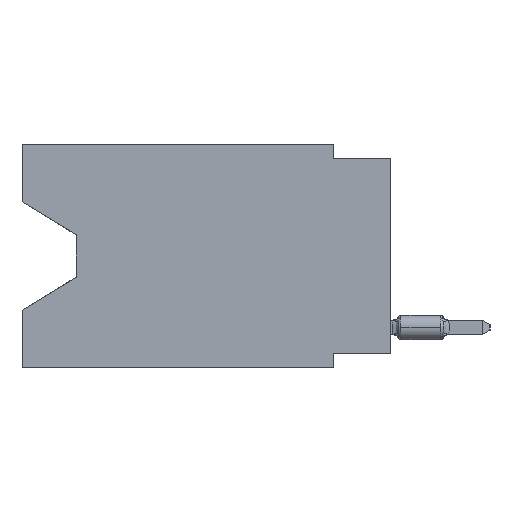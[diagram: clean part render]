
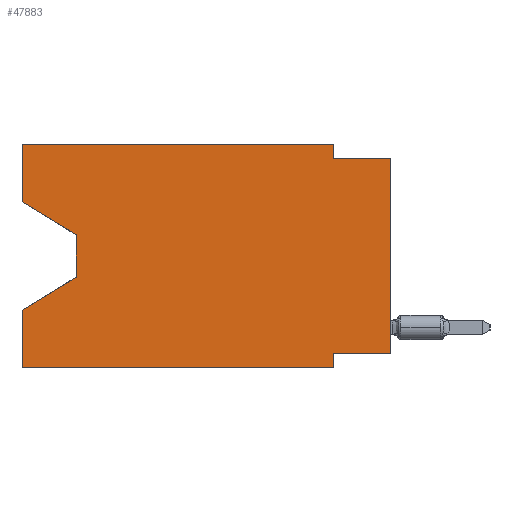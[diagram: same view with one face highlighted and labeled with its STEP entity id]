
A CAD part, left-side view. The second image highlights one B-rep face of the part: STEP entity #47883.
In plain terms, the highlighted planar face has unit normal (-1, 0, 0).
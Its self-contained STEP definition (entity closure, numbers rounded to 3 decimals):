
#1204 = CARTESIAN_POINT ( 'NONE',  ( 0., 16.383, -2.546 ) ) ;
#3223 = CARTESIAN_POINT ( 'NONE',  ( 0., 16.383, -9.906 ) ) ;
#3280 = ORIENTED_EDGE ( 'NONE', *, *, #9359, .F. ) ;
#3339 = CARTESIAN_POINT ( 'NONE',  ( 0., 16.383, 0. ) ) ;
#3977 = VERTEX_POINT ( 'NONE', #37726 ) ;
#4038 = CARTESIAN_POINT ( 'NONE',  ( 0., 0., -0.635 ) ) ;
#4689 = ORIENTED_EDGE ( 'NONE', *, *, #19832, .F. ) ;
#5137 = LINE ( 'NONE', #14670, #37281 ) ;
#5842 = AXIS2_PLACEMENT_3D ( 'NONE', #3339, #15400, #18694 ) ;
#6745 = VECTOR ( 'NONE', #31035, 1000. ) ;
#6858 = CARTESIAN_POINT ( 'NONE',  ( 0., 16.383, 0. ) ) ;
#7104 = DIRECTION ( 'NONE',  ( 0., -1., 0. ) ) ;
#7343 = LINE ( 'NONE', #22481, #6745 ) ;
#8064 = VECTOR ( 'NONE', #26135, 1000. ) ;
#8374 = EDGE_CURVE ( 'NONE', #20429, #22613, #20803, .T. ) ;
#8928 = EDGE_CURVE ( 'NONE', #46024, #38922, #5137, .T. ) ;
#9132 = EDGE_CURVE ( 'NONE', #48511, #3977, #7343, .T. ) ;
#9359 = EDGE_CURVE ( 'NONE', #46024, #48511, #25212, .T. ) ;
#10080 = EDGE_CURVE ( 'NONE', #17925, #31157, #37848, .T. ) ;
#11114 = FACE_OUTER_BOUND ( 'NONE', #37714, .T. ) ;
#11973 = CARTESIAN_POINT ( 'NONE',  ( 0., 16.383, -2.546 ) ) ;
#12024 = LINE ( 'NONE', #38232, #37107 ) ;
#12981 = CARTESIAN_POINT ( 'NONE',  ( 0., 16.383, -9.906 ) ) ;
#13785 = LINE ( 'NONE', #40510, #45194 ) ;
#14670 = CARTESIAN_POINT ( 'NONE',  ( 0., 0., 0. ) ) ;
#15400 = DIRECTION ( 'NONE',  ( 1., 0., 0. ) ) ;
#15571 = CARTESIAN_POINT ( 'NONE',  ( 0., 16.383, 0. ) ) ;
#15615 = ORIENTED_EDGE ( 'NONE', *, *, #24946, .F. ) ;
#17768 = LINE ( 'NONE', #21801, #44777 ) ;
#17925 = VERTEX_POINT ( 'NONE', #43346 ) ;
#17985 = ORIENTED_EDGE ( 'NONE', *, *, #48551, .T. ) ;
#18386 = ORIENTED_EDGE ( 'NONE', *, *, #9132, .F. ) ;
#18694 = DIRECTION ( 'NONE',  ( 0., 0., -1. ) ) ;
#18767 = VECTOR ( 'NONE', #47257, 1000. ) ;
#18847 = DIRECTION ( 'NONE',  ( 0., 0., 1. ) ) ;
#19832 = EDGE_CURVE ( 'NONE', #28555, #35747, #12024, .T. ) ;
#20429 = VERTEX_POINT ( 'NONE', #11973 ) ;
#20803 = LINE ( 'NONE', #1204, #18767 ) ;
#21218 = ORIENTED_EDGE ( 'NONE', *, *, #31844, .T. ) ;
#21319 = CARTESIAN_POINT ( 'NONE',  ( 0., 0., -0.635 ) ) ;
#21801 = CARTESIAN_POINT ( 'NONE',  ( 0., 2.54, 0. ) ) ;
#21937 = DIRECTION ( 'NONE',  ( 0., 1., 0. ) ) ;
#22116 = ORIENTED_EDGE ( 'NONE', *, *, #36524, .T. ) ;
#22481 = CARTESIAN_POINT ( 'NONE',  ( 0., 2.54, -9.906 ) ) ;
#22613 = VERTEX_POINT ( 'NONE', #39816 ) ;
#22615 = LINE ( 'NONE', #37974, #8064 ) ;
#24548 = VERTEX_POINT ( 'NONE', #49396 ) ;
#24885 = CARTESIAN_POINT ( 'NONE',  ( 0., 2.54, 0. ) ) ;
#24946 = EDGE_CURVE ( 'NONE', #20429, #17925, #37999, .T. ) ;
#25212 = LINE ( 'NONE', #40587, #38139 ) ;
#25267 = DIRECTION ( 'NONE',  ( 0., 0., 1. ) ) ;
#26135 = DIRECTION ( 'NONE',  ( 0., 0.855, -0.519 ) ) ;
#26741 = PLANE ( 'NONE',  #5842 ) ;
#27827 = DIRECTION ( 'NONE',  ( 0., 0., 1. ) ) ;
#28160 = DIRECTION ( 'NONE',  ( 0., 0., -1. ) ) ;
#28222 = VECTOR ( 'NONE', #48020, 1000. ) ;
#28357 = DIRECTION ( 'NONE',  ( 0., -1., 0. ) ) ;
#28472 = CARTESIAN_POINT ( 'NONE',  ( 0., 16.383, -7.36 ) ) ;
#28555 = VERTEX_POINT ( 'NONE', #3223 ) ;
#28644 = VECTOR ( 'NONE', #28357, 1000. ) ;
#30017 = EDGE_CURVE ( 'NONE', #31284, #38922, #48263, .T. ) ;
#31035 = DIRECTION ( 'NONE',  ( 0., 0., -1. ) ) ;
#31157 = VERTEX_POINT ( 'NONE', #24885 ) ;
#31284 = VERTEX_POINT ( 'NONE', #45287 ) ;
#31829 = ORIENTED_EDGE ( 'NONE', *, *, #30017, .F. ) ;
#31844 = EDGE_CURVE ( 'NONE', #24548, #35747, #22615, .T. ) ;
#33018 = ORIENTED_EDGE ( 'NONE', *, *, #8928, .T. ) ;
#35091 = CARTESIAN_POINT ( 'NONE',  ( 0., 0., -9.271 ) ) ;
#35747 = VERTEX_POINT ( 'NONE', #28472 ) ;
#36524 = EDGE_CURVE ( 'NONE', #28555, #3977, #43000, .T. ) ;
#36710 = EDGE_CURVE ( 'NONE', #31157, #31284, #17768, .T. ) ;
#36860 = ORIENTED_EDGE ( 'NONE', *, *, #36710, .F. ) ;
#37107 = VECTOR ( 'NONE', #18847, 1000. ) ;
#37146 = VECTOR ( 'NONE', #7104, 1000. ) ;
#37281 = VECTOR ( 'NONE', #25267, 1000. ) ;
#37714 = EDGE_LOOP ( 'NONE', ( #48249, #17985, #21218, #4689, #22116, #18386, #3280, #33018, #31829, #36860, #40764, #15615 ) ) ;
#37726 = CARTESIAN_POINT ( 'NONE',  ( 0., 2.54, -9.906 ) ) ;
#37848 = LINE ( 'NONE', #6858, #37146 ) ;
#37974 = CARTESIAN_POINT ( 'NONE',  ( 0., 13.97, -5.893 ) ) ;
#37999 = LINE ( 'NONE', #15571, #47140 ) ;
#38139 = VECTOR ( 'NONE', #21937, 1000. ) ;
#38232 = CARTESIAN_POINT ( 'NONE',  ( 0., 16.383, 0. ) ) ;
#38922 = VERTEX_POINT ( 'NONE', #4038 ) ;
#39816 = CARTESIAN_POINT ( 'NONE',  ( 0., 13.97, -4.013 ) ) ;
#40510 = CARTESIAN_POINT ( 'NONE',  ( 0., 13.97, -4.013 ) ) ;
#40587 = CARTESIAN_POINT ( 'NONE',  ( 0., 0., -9.271 ) ) ;
#40764 = ORIENTED_EDGE ( 'NONE', *, *, #10080, .F. ) ;
#43000 = LINE ( 'NONE', #12981, #28644 ) ;
#43346 = CARTESIAN_POINT ( 'NONE',  ( 0., 16.383, 0. ) ) ;
#44229 = DIRECTION ( 'NONE',  ( 0., 0., -1. ) ) ;
#44777 = VECTOR ( 'NONE', #44229, 1000. ) ;
#45194 = VECTOR ( 'NONE', #28160, 1000. ) ;
#45287 = CARTESIAN_POINT ( 'NONE',  ( 0., 2.54, -0.635 ) ) ;
#46024 = VERTEX_POINT ( 'NONE', #35091 ) ;
#47140 = VECTOR ( 'NONE', #27827, 1000. ) ;
#47257 = DIRECTION ( 'NONE',  ( 0., -0.855, -0.519 ) ) ;
#47883 = ADVANCED_FACE ( 'NONE', ( #11114 ), #26741, .F. ) ;
#48020 = DIRECTION ( 'NONE',  ( 0., -1., 0. ) ) ;
#48051 = CARTESIAN_POINT ( 'NONE',  ( 0., 2.54, -9.271 ) ) ;
#48249 = ORIENTED_EDGE ( 'NONE', *, *, #8374, .T. ) ;
#48263 = LINE ( 'NONE', #21319, #28222 ) ;
#48511 = VERTEX_POINT ( 'NONE', #48051 ) ;
#48551 = EDGE_CURVE ( 'NONE', #22613, #24548, #13785, .T. ) ;
#49396 = CARTESIAN_POINT ( 'NONE',  ( 0., 13.97, -5.893 ) ) ;
